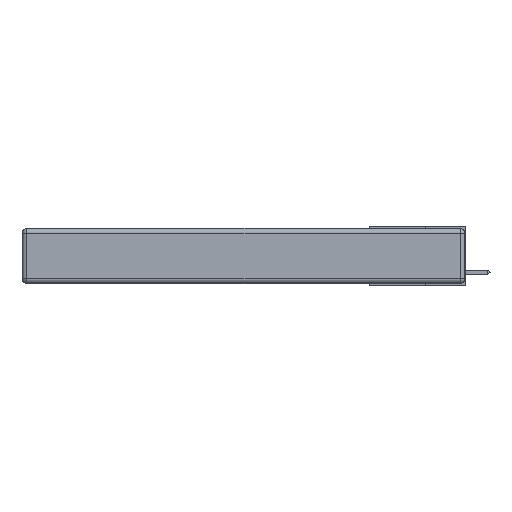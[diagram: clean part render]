
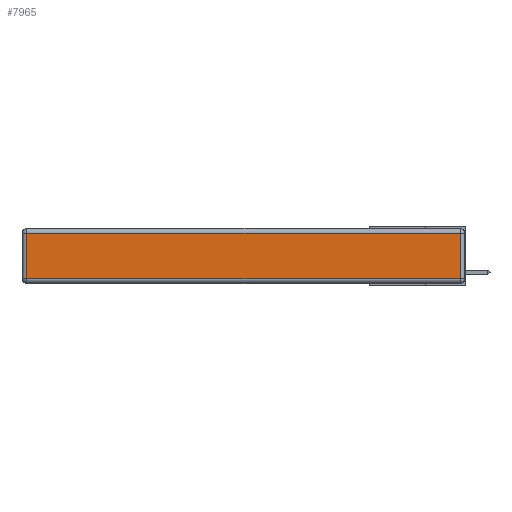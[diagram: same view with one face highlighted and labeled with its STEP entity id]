
A CAD part, left-side view. The second image highlights one B-rep face of the part: STEP entity #7965.
In plain terms, the highlighted planar face has unit normal (-1, 0, 0).
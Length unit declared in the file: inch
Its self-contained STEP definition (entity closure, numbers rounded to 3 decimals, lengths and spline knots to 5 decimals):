
#595 = VECTOR ( 'NONE', #21906, 39.37008 ) ;
#711 = FACE_OUTER_BOUND ( 'NONE', #16544, .T. ) ;
#2415 = LINE ( 'NONE', #24733, #22908 ) ;
#4349 = LINE ( 'NONE', #13852, #595 ) ;
#5450 = VERTEX_POINT ( 'NONE', #26206 ) ;
#5508 = ORIENTED_EDGE ( 'NONE', *, *, #33973, .T. ) ;
#6511 = LINE ( 'NONE', #13866, #22806 ) ;
#7503 = PLANE ( 'NONE',  #30100 ) ;
#7965 = ADVANCED_FACE ( 'NONE', ( #711 ), #7503, .T. ) ;
#8559 = LINE ( 'NONE', #30781, #19452 ) ;
#10388 = EDGE_CURVE ( 'NONE', #31784, #5450, #8559, .T. ) ;
#12231 = ORIENTED_EDGE ( 'NONE', *, *, #22048, .T. ) ;
#13457 = CARTESIAN_POINT ( 'NONE',  ( 0., 0.03, -0.03 ) ) ;
#13852 = CARTESIAN_POINT ( 'NONE',  ( 0., 0.03, -0.343 ) ) ;
#13866 = CARTESIAN_POINT ( 'NONE',  ( 0., 2.72, -0.343 ) ) ;
#13867 = CARTESIAN_POINT ( 'NONE',  ( 0., 0.03, -0.313 ) ) ;
#14596 = EDGE_CURVE ( 'NONE', #5450, #31583, #6511, .T. ) ;
#14853 = DIRECTION ( 'NONE',  ( 0., 1., 0. ) ) ;
#14967 = CARTESIAN_POINT ( 'NONE',  ( 0., 0., -0.343 ) ) ;
#16544 = EDGE_LOOP ( 'NONE', ( #12231, #5508, #22476, #16851 ) ) ;
#16851 = ORIENTED_EDGE ( 'NONE', *, *, #14596, .T. ) ;
#17079 = VERTEX_POINT ( 'NONE', #13867 ) ;
#19452 = VECTOR ( 'NONE', #14853, 39.37008 ) ;
#21906 = DIRECTION ( 'NONE',  ( 0., 0., 1. ) ) ;
#22048 = EDGE_CURVE ( 'NONE', #31583, #17079, #2415, .T. ) ;
#22476 = ORIENTED_EDGE ( 'NONE', *, *, #10388, .T. ) ;
#22806 = VECTOR ( 'NONE', #30146, 39.37008 ) ;
#22908 = VECTOR ( 'NONE', #32829, 39.37008 ) ;
#24733 = CARTESIAN_POINT ( 'NONE',  ( 0., 0., -0.313 ) ) ;
#26036 = DIRECTION ( 'NONE',  ( 0., 0., 1. ) ) ;
#26206 = CARTESIAN_POINT ( 'NONE',  ( 0., 2.72, -0.03 ) ) ;
#30100 = AXIS2_PLACEMENT_3D ( 'NONE', #14967, #31028, #26036 ) ;
#30146 = DIRECTION ( 'NONE',  ( 0., 0., -1. ) ) ;
#30781 = CARTESIAN_POINT ( 'NONE',  ( 0., 2.75, -0.03 ) ) ;
#31028 = DIRECTION ( 'NONE',  ( -1., 0., 0. ) ) ;
#31438 = CARTESIAN_POINT ( 'NONE',  ( 0., 2.72, -0.313 ) ) ;
#31583 = VERTEX_POINT ( 'NONE', #31438 ) ;
#31784 = VERTEX_POINT ( 'NONE', #13457 ) ;
#32829 = DIRECTION ( 'NONE',  ( 0., -1., 0. ) ) ;
#33973 = EDGE_CURVE ( 'NONE', #17079, #31784, #4349, .T. ) ;
